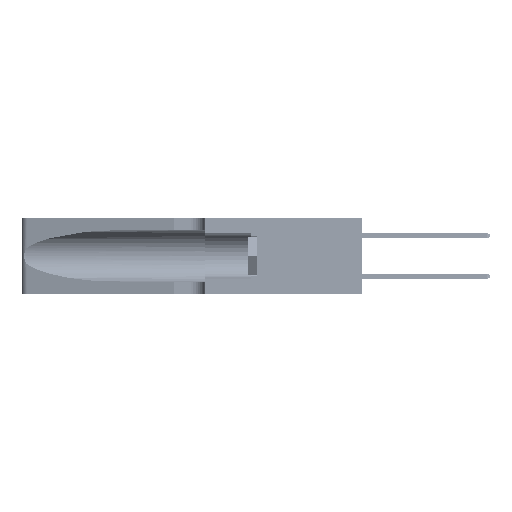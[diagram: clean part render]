
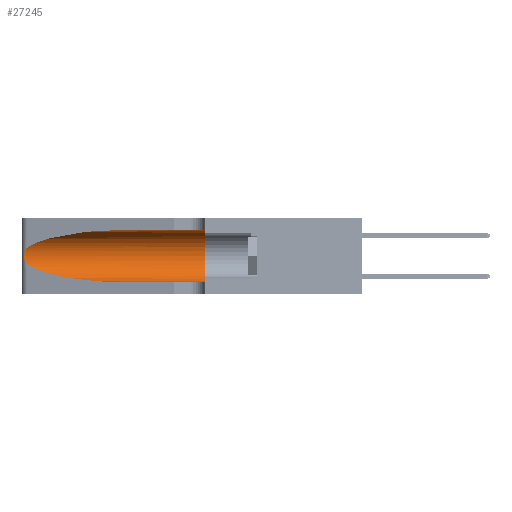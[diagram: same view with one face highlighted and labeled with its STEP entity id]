
A CAD part, left-side view. The second image highlights one B-rep face of the part: STEP entity #27245.
In plain terms, the highlighted cylindrical face has radius 3.308 mm (diameter 6.617 mm), a partial arc.
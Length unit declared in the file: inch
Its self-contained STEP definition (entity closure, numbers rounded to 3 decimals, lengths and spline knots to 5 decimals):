
#24 = CARTESIAN_POINT ( 'NONE',  ( 0.1305, 1.61858, 0.05475 ) ) ;
#507 = CARTESIAN_POINT ( 'NONE',  ( 0.26017, 1.23833, 0.17102 ) ) ;
#513 = CARTESIAN_POINT ( 'NONE',  ( 0.25487, 1.22718, 0.22369 ) ) ;
#780 = CARTESIAN_POINT ( 'NONE',  ( 0.25487, 1.22718, 0.14631 ) ) ;
#1803 = DIRECTION ( 'NONE',  ( 0., -1., 0. ) ) ;
#2507 = FACE_OUTER_BOUND ( 'NONE', #28170, .T. ) ;
#3780 = VERTEX_POINT ( 'NONE', #21495 ) ;
#4810 = CARTESIAN_POINT ( 'NONE',  ( 0.25487, 1.22718, 0.22369 ) ) ;
#5757 = ORIENTED_EDGE ( 'NONE', *, *, #14270, .T. ) ;
#5909 = VERTEX_POINT ( 'NONE', #19007 ) ;
#6890 = CARTESIAN_POINT ( 'NONE',  ( 0.25854, 1.2359, 0.20912 ) ) ;
#7616 =( BOUNDED_CURVE ( )  B_SPLINE_CURVE ( 3, ( #780, #39135, #23940, #27910 ),
 .UNSPECIFIED., .F., .F. ) 
 B_SPLINE_CURVE_WITH_KNOTS ( ( 4, 4 ),
 ( 3.44316, 4.71239 ),
 .UNSPECIFIED. ) 
 CURVE ( )  GEOMETRIC_REPRESENTATION_ITEM ( )  RATIONAL_B_SPLINE_CURVE ( ( 1., 0.87, 0.87, 1. ) ) 
 REPRESENTATION_ITEM ( '' )  );
#7819 = CYLINDRICAL_SURFACE ( 'NONE', #45767, 0.13025 ) ;
#8114 = CARTESIAN_POINT ( 'NONE',  ( 0.25856, 1.23593, 0.16098 ) ) ;
#9319 = CARTESIAN_POINT ( 'NONE',  ( 0.1305, 1.61858, 0.185 ) ) ;
#9916 = VECTOR ( 'NONE', #1803, 39.37008 ) ;
#10874 = DIRECTION ( 'NONE',  ( 0., 1., 0. ) ) ;
#12643 = ORIENTED_EDGE ( 'NONE', *, *, #46759, .F. ) ;
#13220 = EDGE_CURVE ( 'NONE', #15169, #40200, #7616, .T. ) ;
#13525 = CARTESIAN_POINT ( 'NONE',  ( 0.1305, 0.72297, 0.05475 ) ) ;
#14270 = EDGE_CURVE ( 'NONE', #5909, #38193, #45781, .T. ) ;
#15062 = CARTESIAN_POINT ( 'NONE',  ( 0.26018, 1.23835, 0.19895 ) ) ;
#15169 = VERTEX_POINT ( 'NONE', #27244 ) ;
#15317 = CIRCLE ( 'NONE', #37634, 0.13025 ) ;
#15654 = ORIENTED_EDGE ( 'NONE', *, *, #42340, .F. ) ;
#17900 = CARTESIAN_POINT ( 'NONE',  ( 0.25487, 1.22718, 0.22369 ) ) ;
#19007 = CARTESIAN_POINT ( 'NONE',  ( 0.1305, 0.72297, 0.31525 ) ) ;
#19025 = CARTESIAN_POINT ( 'NONE',  ( 0.25555, 1.22993, 0.14849 ) ) ;
#19988 = LINE ( 'NONE', #46756, #9916 ) ;
#20365 = VECTOR ( 'NONE', #48934, 39.37008 ) ;
#21398 = DIRECTION ( 'NONE',  ( 0., -1., 0. ) ) ;
#21495 = CARTESIAN_POINT ( 'NONE',  ( 0.1305, 0.35, 0.05475 ) ) ;
#22288 = DIRECTION ( 'NONE',  ( 0., 0., 1. ) ) ;
#23548 = CARTESIAN_POINT ( 'NONE',  ( 0.25639, 1.23184, 0.21858 ) ) ;
#23940 = CARTESIAN_POINT ( 'NONE',  ( 0.18966, 0.96281, 0.05475 ) ) ;
#24765 = ORIENTED_EDGE ( 'NONE', *, *, #13220, .T. ) ;
#25638 = EDGE_CURVE ( 'NONE', #40200, #3780, #42265, .T. ) ;
#26318 = CARTESIAN_POINT ( 'NONE',  ( 0.26075, 1.23896, 0.178 ) ) ;
#26654 = CARTESIAN_POINT ( 'NONE',  ( 0.25487, 1.22718, 0.14631 ) ) ;
#27244 = CARTESIAN_POINT ( 'NONE',  ( 0.25487, 1.22718, 0.14631 ) ) ;
#27245 = ADVANCED_FACE ( 'NONE', ( #2507 ), #7819, .F. ) ;
#27910 = CARTESIAN_POINT ( 'NONE',  ( 0.1305, 0.72297, 0.05475 ) ) ;
#28170 = EDGE_LOOP ( 'NONE', ( #5757, #45478, #24765, #33877, #12643, #15654 ) ) ;
#30803 = CARTESIAN_POINT ( 'NONE',  ( 0.1305, 0.35, 0.31525 ) ) ;
#32351 = DIRECTION ( 'NONE',  ( 0., 0., -1. ) ) ;
#33769 = CARTESIAN_POINT ( 'NONE',  ( 0.2373, 1.15595, 0.28018 ) ) ;
#33877 = ORIENTED_EDGE ( 'NONE', *, *, #25638, .T. ) ;
#34427 = CARTESIAN_POINT ( 'NONE',  ( 0.25639, 1.23186, 0.15144 ) ) ;
#37634 = AXIS2_PLACEMENT_3D ( 'NONE', #44929, #10874, #22288 ) ;
#38193 = VERTEX_POINT ( 'NONE', #4810 ) ;
#38373 = CARTESIAN_POINT ( 'NONE',  ( 0.25787, 1.23484, 0.2124 ) ) ;
#39135 = CARTESIAN_POINT ( 'NONE',  ( 0.2373, 1.15595, 0.08982 ) ) ;
#40200 = VERTEX_POINT ( 'NONE', #13525 ) ;
#41665 = CARTESIAN_POINT ( 'NONE',  ( 0.18966, 0.96281, 0.31525 ) ) ;
#41675 = CARTESIAN_POINT ( 'NONE',  ( 0.26075, 1.23896, 0.19203 ) ) ;
#41839 = CARTESIAN_POINT ( 'NONE',  ( 0.25789, 1.23486, 0.15765 ) ) ;
#42265 = LINE ( 'NONE', #24, #20365 ) ;
#42340 = EDGE_CURVE ( 'NONE', #5909, #48197, #19988, .T. ) ;
#44356 = CARTESIAN_POINT ( 'NONE',  ( 0.25555, 1.22994, 0.2215 ) ) ;
#44929 = CARTESIAN_POINT ( 'NONE',  ( 0.1305, 0.35, 0.185 ) ) ;
#44977 = CARTESIAN_POINT ( 'NONE',  ( 0.1305, 0.72297, 0.31525 ) ) ;
#45478 = ORIENTED_EDGE ( 'NONE', *, *, #46186, .T. ) ;
#45767 = AXIS2_PLACEMENT_3D ( 'NONE', #9319, #21398, #32351 ) ;
#45781 =( BOUNDED_CURVE ( )  B_SPLINE_CURVE ( 3, ( #44977, #41665, #33769, #513 ),
 .UNSPECIFIED., .F., .F. ) 
 B_SPLINE_CURVE_WITH_KNOTS ( ( 4, 4 ),
 ( 1.5708, 2.84003 ),
 .UNSPECIFIED. ) 
 CURVE ( )  GEOMETRIC_REPRESENTATION_ITEM ( )  RATIONAL_B_SPLINE_CURVE ( ( 1., 0.87, 0.87, 1. ) ) 
 REPRESENTATION_ITEM ( '' )  );
#46186 = EDGE_CURVE ( 'NONE', #38193, #15169, #48511, .T. ) ;
#46756 = CARTESIAN_POINT ( 'NONE',  ( 0.1305, 1.61858, 0.31525 ) ) ;
#46759 = EDGE_CURVE ( 'NONE', #48197, #3780, #15317, .T. ) ;
#48197 = VERTEX_POINT ( 'NONE', #30803 ) ;
#48511 = B_SPLINE_CURVE_WITH_KNOTS ( 'NONE', 3,
 ( #17900, #44356, #23548, #38373, #6890, #15062, #41675, #26318, #507, #8114, #41839, #34427, #19025, #26654 ),
 .UNSPECIFIED., .F., .F.,
 ( 4, 2, 2, 2, 2, 2, 4 ),
 ( 0., 0.00027, 0.00053, 0.00107, 0.0016, 0.00187, 0.00214 ),
 .UNSPECIFIED. ) ;
#48934 = DIRECTION ( 'NONE',  ( 0., -1., 0. ) ) ;
